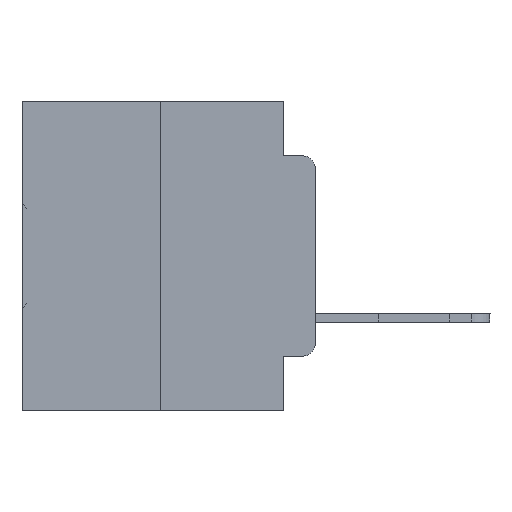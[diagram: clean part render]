
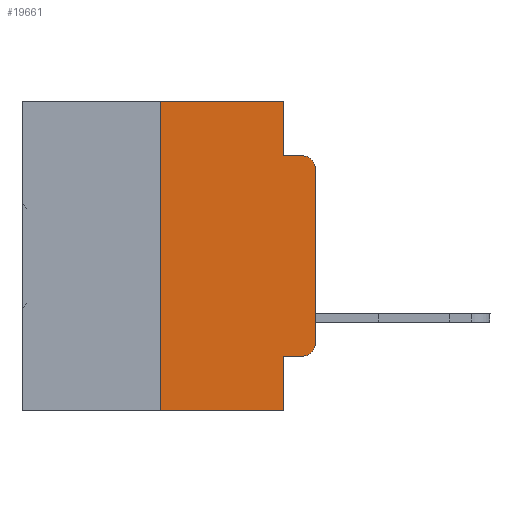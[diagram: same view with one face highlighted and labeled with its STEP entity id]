
A CAD part, left-side view. The second image highlights one B-rep face of the part: STEP entity #19661.
In plain terms, the highlighted planar face has unit normal (-1, 0, 0).
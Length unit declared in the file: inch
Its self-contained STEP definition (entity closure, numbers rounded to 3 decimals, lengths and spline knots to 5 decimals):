
#281 = DIRECTION ( 'NONE',  ( 0., 0., 1. ) ) ;
#1051 = AXIS2_PLACEMENT_3D ( 'NONE', #1570, #30450, #7047 ) ;
#1141 = CIRCLE ( 'NONE', #3894, 0.02 ) ;
#1148 = EDGE_CURVE ( 'NONE', #19760, #6655, #16003, .T. ) ;
#1316 = EDGE_LOOP ( 'NONE', ( #20320, #24557, #25909, #9466, #24760, #27320, #13576, #13806, #14625, #29585 ) ) ;
#1336 = DIRECTION ( 'NONE',  ( 0., 0., -1. ) ) ;
#1570 = CARTESIAN_POINT ( 'NONE',  ( 0., 0.02, -0.3915 ) ) ;
#1747 = DIRECTION ( 'NONE',  ( 0., 0., -1. ) ) ;
#2839 = DIRECTION ( 'NONE',  ( 0., 0., -1. ) ) ;
#3089 = LINE ( 'NONE', #11115, #28879 ) ;
#3143 = EDGE_CURVE ( 'NONE', #20218, #14052, #1141, .T. ) ;
#3894 = AXIS2_PLACEMENT_3D ( 'NONE', #30295, #33184, #1747 ) ;
#3914 = LINE ( 'NONE', #24761, #30129 ) ;
#4348 = EDGE_CURVE ( 'NONE', #21746, #20218, #17575, .T. ) ;
#4737 = CARTESIAN_POINT ( 'NONE',  ( 0., 0., -0.1085 ) ) ;
#4785 = VERTEX_POINT ( 'NONE', #22147 ) ;
#5455 = CARTESIAN_POINT ( 'NONE',  ( 0., 0.051, 0. ) ) ;
#5939 = LINE ( 'NONE', #23713, #27962 ) ;
#6087 = AXIS2_PLACEMENT_3D ( 'NONE', #19995, #16929, #14700 ) ;
#6655 = VERTEX_POINT ( 'NONE', #21911 ) ;
#7047 = DIRECTION ( 'NONE',  ( 0., 0., -1. ) ) ;
#8049 = DIRECTION ( 'NONE',  ( 0., -1., 0. ) ) ;
#8700 = CIRCLE ( 'NONE', #1051, 0.02 ) ;
#9263 = EDGE_CURVE ( 'NONE', #4785, #18203, #12095, .T. ) ;
#9300 = EDGE_CURVE ( 'NONE', #6655, #14052, #29710, .T. ) ;
#9466 = ORIENTED_EDGE ( 'NONE', *, *, #1148, .F. ) ;
#9701 = DIRECTION ( 'NONE',  ( 0., 0., 1. ) ) ;
#11016 = VERTEX_POINT ( 'NONE', #14250 ) ;
#11115 = CARTESIAN_POINT ( 'NONE',  ( 0., 0.473, 0. ) ) ;
#11583 = DIRECTION ( 'NONE',  ( 0., -1., 0. ) ) ;
#11826 = CARTESIAN_POINT ( 'NONE',  ( 0., 0.051, -0.5 ) ) ;
#11936 = CARTESIAN_POINT ( 'NONE',  ( 0., 0., 0. ) ) ;
#12095 = LINE ( 'NONE', #17051, #18350 ) ;
#12309 = FACE_OUTER_BOUND ( 'NONE', #1316, .T. ) ;
#13576 = ORIENTED_EDGE ( 'NONE', *, *, #25007, .T. ) ;
#13806 = ORIENTED_EDGE ( 'NONE', *, *, #21007, .F. ) ;
#14052 = VERTEX_POINT ( 'NONE', #20112 ) ;
#14250 = CARTESIAN_POINT ( 'NONE',  ( 0., 0.25, 0. ) ) ;
#14625 = ORIENTED_EDGE ( 'NONE', *, *, #9263, .T. ) ;
#14700 = DIRECTION ( 'NONE',  ( 0., 0., -1. ) ) ;
#15606 = DIRECTION ( 'NONE',  ( 0., -1., 0. ) ) ;
#16003 = LINE ( 'NONE', #33757, #19425 ) ;
#16929 = DIRECTION ( 'NONE',  ( 1., 0., 0. ) ) ;
#17051 = CARTESIAN_POINT ( 'NONE',  ( 0., 0.051, -0.4115 ) ) ;
#17575 = LINE ( 'NONE', #11936, #21422 ) ;
#17961 = EDGE_CURVE ( 'NONE', #18203, #21746, #8700, .T. ) ;
#18000 = CARTESIAN_POINT ( 'NONE',  ( 0., 0.473, -0.5 ) ) ;
#18203 = VERTEX_POINT ( 'NONE', #19332 ) ;
#18350 = VECTOR ( 'NONE', #11583, 39.37008 ) ;
#19332 = CARTESIAN_POINT ( 'NONE',  ( 0., 0.02, -0.4115 ) ) ;
#19425 = VECTOR ( 'NONE', #2839, 39.37008 ) ;
#19661 = ADVANCED_FACE ( 'NONE', ( #12309 ), #30080, .F. ) ;
#19760 = VERTEX_POINT ( 'NONE', #5455 ) ;
#19995 = CARTESIAN_POINT ( 'NONE',  ( 0., 0.473, 0. ) ) ;
#20112 = CARTESIAN_POINT ( 'NONE',  ( 0., 0.02, -0.0885 ) ) ;
#20218 = VERTEX_POINT ( 'NONE', #4737 ) ;
#20320 = ORIENTED_EDGE ( 'NONE', *, *, #4348, .T. ) ;
#21007 = EDGE_CURVE ( 'NONE', #4785, #32064, #3914, .T. ) ;
#21153 = VECTOR ( 'NONE', #15606, 39.37008 ) ;
#21422 = VECTOR ( 'NONE', #9701, 39.37008 ) ;
#21746 = VERTEX_POINT ( 'NONE', #25142 ) ;
#21860 = VERTEX_POINT ( 'NONE', #27873 ) ;
#21911 = CARTESIAN_POINT ( 'NONE',  ( 0., 0.051, -0.0885 ) ) ;
#22147 = CARTESIAN_POINT ( 'NONE',  ( 0., 0.051, -0.4115 ) ) ;
#22498 = EDGE_CURVE ( 'NONE', #21860, #11016, #5939, .T. ) ;
#22689 = CARTESIAN_POINT ( 'NONE',  ( 0., 0.051, -0.0885 ) ) ;
#23713 = CARTESIAN_POINT ( 'NONE',  ( 0., 0.25, 0. ) ) ;
#24557 = ORIENTED_EDGE ( 'NONE', *, *, #3143, .T. ) ;
#24760 = ORIENTED_EDGE ( 'NONE', *, *, #26803, .F. ) ;
#24761 = CARTESIAN_POINT ( 'NONE',  ( 0., 0.051, 0. ) ) ;
#25007 = EDGE_CURVE ( 'NONE', #21860, #32064, #33199, .T. ) ;
#25142 = CARTESIAN_POINT ( 'NONE',  ( 0., 0., -0.3915 ) ) ;
#25909 = ORIENTED_EDGE ( 'NONE', *, *, #9300, .F. ) ;
#26803 = EDGE_CURVE ( 'NONE', #11016, #19760, #3089, .T. ) ;
#27320 = ORIENTED_EDGE ( 'NONE', *, *, #22498, .F. ) ;
#27873 = CARTESIAN_POINT ( 'NONE',  ( 0., 0.25, -0.5 ) ) ;
#27962 = VECTOR ( 'NONE', #281, 39.37008 ) ;
#28879 = VECTOR ( 'NONE', #8049, 39.37008 ) ;
#29585 = ORIENTED_EDGE ( 'NONE', *, *, #17961, .T. ) ;
#29710 = LINE ( 'NONE', #22689, #31408 ) ;
#30080 = PLANE ( 'NONE',  #6087 ) ;
#30129 = VECTOR ( 'NONE', #1336, 39.37008 ) ;
#30295 = CARTESIAN_POINT ( 'NONE',  ( 0., 0.02, -0.1085 ) ) ;
#30450 = DIRECTION ( 'NONE',  ( -1., 0., 0. ) ) ;
#31408 = VECTOR ( 'NONE', #33093, 39.37008 ) ;
#32064 = VERTEX_POINT ( 'NONE', #11826 ) ;
#33093 = DIRECTION ( 'NONE',  ( 0., -1., 0. ) ) ;
#33184 = DIRECTION ( 'NONE',  ( -1., 0., 0. ) ) ;
#33199 = LINE ( 'NONE', #18000, #21153 ) ;
#33757 = CARTESIAN_POINT ( 'NONE',  ( 0., 0.051, 0. ) ) ;
